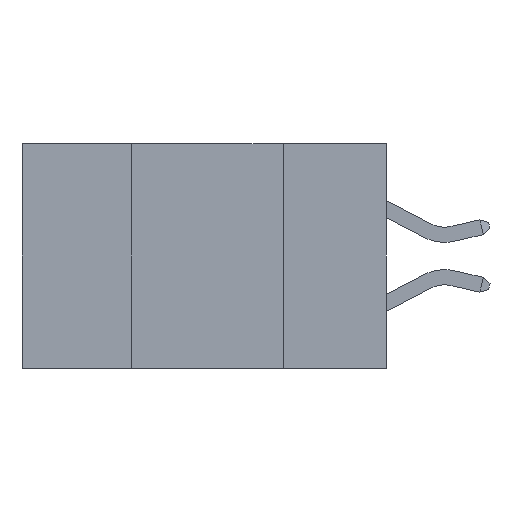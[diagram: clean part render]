
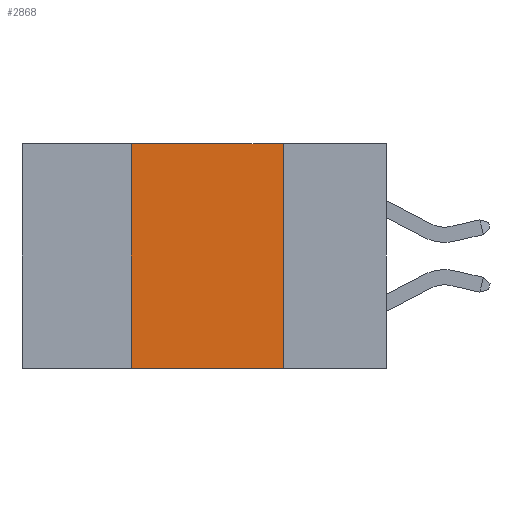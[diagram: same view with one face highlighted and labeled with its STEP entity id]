
A CAD part, left-side view. The second image highlights one B-rep face of the part: STEP entity #2868.
In plain terms, the highlighted planar face has unit normal (-1, 0, 0).
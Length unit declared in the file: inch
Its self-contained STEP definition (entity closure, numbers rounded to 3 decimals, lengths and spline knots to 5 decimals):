
#6 = DIRECTION ( 'NONE',  ( 0., 0., -1. ) ) ;
#432 = CARTESIAN_POINT ( 'NONE',  ( 0., 0.42, -0.37 ) ) ;
#1003 = EDGE_LOOP ( 'NONE', ( #3938, #9693, #8249, #10483 ) ) ;
#1446 = CARTESIAN_POINT ( 'NONE',  ( 0., 0.17, 0. ) ) ;
#1451 = DIRECTION ( 'NONE',  ( 0., 0., 1. ) ) ;
#2052 = LINE ( 'NONE', #6059, #9570 ) ;
#2431 = VERTEX_POINT ( 'NONE', #6493 ) ;
#2747 = VECTOR ( 'NONE', #1451, 39.37008 ) ;
#2868 = ADVANCED_FACE ( 'NONE', ( #5839 ), #5085, .F. ) ;
#3012 = EDGE_CURVE ( 'NONE', #3280, #2431, #5983, .T. ) ;
#3066 = LINE ( 'NONE', #432, #2747 ) ;
#3280 = VERTEX_POINT ( 'NONE', #12838 ) ;
#3453 = EDGE_CURVE ( 'NONE', #6368, #2431, #5833, .T. ) ;
#3938 = ORIENTED_EDGE ( 'NONE', *, *, #3453, .F. ) ;
#4383 = EDGE_CURVE ( 'NONE', #3280, #9059, #3066, .T. ) ;
#5085 = PLANE ( 'NONE',  #6023 ) ;
#5833 = LINE ( 'NONE', #10058, #11219 ) ;
#5839 = FACE_OUTER_BOUND ( 'NONE', #1003, .T. ) ;
#5983 = LINE ( 'NONE', #6341, #8369 ) ;
#6023 = AXIS2_PLACEMENT_3D ( 'NONE', #12177, #6124, #6 ) ;
#6059 = CARTESIAN_POINT ( 'NONE',  ( 0., 0.6, 0. ) ) ;
#6124 = DIRECTION ( 'NONE',  ( 1., 0., 0. ) ) ;
#6341 = CARTESIAN_POINT ( 'NONE',  ( 0., 0.6, -0.37 ) ) ;
#6368 = VERTEX_POINT ( 'NONE', #1446 ) ;
#6493 = CARTESIAN_POINT ( 'NONE',  ( 0., 0.17, -0.37 ) ) ;
#6975 = DIRECTION ( 'NONE',  ( 0., 0., -1. ) ) ;
#7067 = DIRECTION ( 'NONE',  ( 0., -1., 0. ) ) ;
#8249 = ORIENTED_EDGE ( 'NONE', *, *, #4383, .F. ) ;
#8369 = VECTOR ( 'NONE', #11401, 39.37008 ) ;
#9059 = VERTEX_POINT ( 'NONE', #9241 ) ;
#9241 = CARTESIAN_POINT ( 'NONE',  ( 0., 0.42, 0. ) ) ;
#9570 = VECTOR ( 'NONE', #7067, 39.37008 ) ;
#9693 = ORIENTED_EDGE ( 'NONE', *, *, #12544, .F. ) ;
#10058 = CARTESIAN_POINT ( 'NONE',  ( 0., 0.17, -0.37 ) ) ;
#10483 = ORIENTED_EDGE ( 'NONE', *, *, #3012, .T. ) ;
#11219 = VECTOR ( 'NONE', #6975, 39.37008 ) ;
#11401 = DIRECTION ( 'NONE',  ( 0., -1., 0. ) ) ;
#12177 = CARTESIAN_POINT ( 'NONE',  ( 0., 0.6, 0. ) ) ;
#12544 = EDGE_CURVE ( 'NONE', #9059, #6368, #2052, .T. ) ;
#12838 = CARTESIAN_POINT ( 'NONE',  ( 0., 0.42, -0.37 ) ) ;
